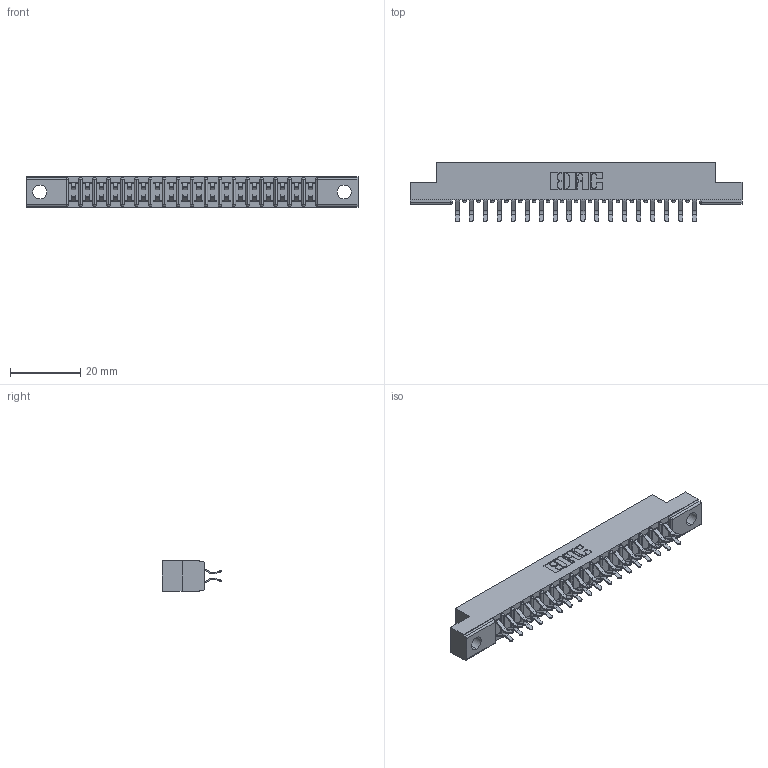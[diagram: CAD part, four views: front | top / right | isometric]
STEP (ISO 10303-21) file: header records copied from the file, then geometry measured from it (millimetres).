
FILE_DESCRIPTION (( 'STEP AP203' ), '1' );
FILE_NAME ('307-036-556-204.STEP', '2019-09-06T03:44:50', ( '' ), ( '' ), 'SwSTEP 2.0', 'SolidWorks 2016', '' );
FILE_SCHEMA (( 'CONFIG_CONTROL_DESIGN' ));
Length unit declared in the file: inch
Products named in the file (3): 307 Part_.156 Dia Mounting Holes; 307-036-556-204; 307-290-001_556
Assembly tree (37 placements, depth 2):
  307-036-556-204
    307 Part_.156 Dia Mounting Holes
    307-290-001_556  x36
Bounding box: 94.34 x 16.97 x 8.71 mm (x, y, z)
Volume: 6058.5 mm3; surface area: 10344.7 mm2
Topology: 37 solids, 37 shells, 1951 faces, 5471 edges, 3546 vertices
Faces by surface type: plane 1272, cylinder 641, sphere 38
Entity records: 19488 total; most frequent: CARTESIAN_POINT 3200, ORIENTED_EDGE 3166, DIRECTION 3137, EDGE_CURVE 1583, VECTOR 1211, LINE 1211, VERTEX_POINT 1026, AXIS2_PLACEMENT_3D 963
